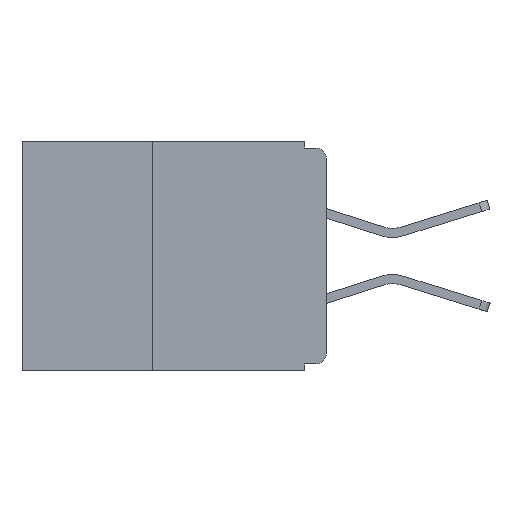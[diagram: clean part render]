
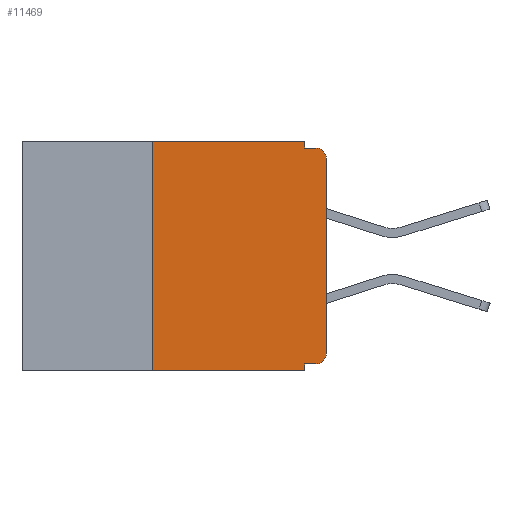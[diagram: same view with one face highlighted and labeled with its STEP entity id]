
A CAD part, left-side view. The second image highlights one B-rep face of the part: STEP entity #11469.
In plain terms, the highlighted planar face has unit normal (-1, 0, 0).
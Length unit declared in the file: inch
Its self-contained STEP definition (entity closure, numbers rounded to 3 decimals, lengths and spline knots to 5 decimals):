
#97 = DIRECTION ( 'NONE',  ( 0., 0., -1. ) ) ;
#202 = VERTEX_POINT ( 'NONE', #6253 ) ;
#437 = ORIENTED_EDGE ( 'NONE', *, *, #6418, .T. ) ;
#735 = ORIENTED_EDGE ( 'NONE', *, *, #865, .F. ) ;
#755 = EDGE_CURVE ( 'NONE', #5003, #202, #6537, .T. ) ;
#865 = EDGE_CURVE ( 'NONE', #6815, #7653, #2872, .T. ) ;
#989 = ORIENTED_EDGE ( 'NONE', *, *, #2569, .F. ) ;
#1243 = DIRECTION ( 'NONE',  ( 0., 0., -1. ) ) ;
#1258 = DIRECTION ( 'NONE',  ( 0., 0., -1. ) ) ;
#1265 = DIRECTION ( 'NONE',  ( -1., 0., 0. ) ) ;
#1297 = CARTESIAN_POINT ( 'NONE',  ( 0., 0.015, -0.305 ) ) ;
#1973 = CARTESIAN_POINT ( 'NONE',  ( 0., 0.031, -0.32 ) ) ;
#2001 = LINE ( 'NONE', #6248, #15230 ) ;
#2160 = CARTESIAN_POINT ( 'NONE',  ( 0., 0., -0.025 ) ) ;
#2253 = VERTEX_POINT ( 'NONE', #12908 ) ;
#2569 = EDGE_CURVE ( 'NONE', #202, #6815, #14484, .T. ) ;
#2672 = DIRECTION ( 'NONE',  ( 0., 0., -1. ) ) ;
#2676 = DIRECTION ( 'NONE',  ( -1., 0., 0. ) ) ;
#2709 = CARTESIAN_POINT ( 'NONE',  ( 0., 0.015, -0.025 ) ) ;
#2716 = VERTEX_POINT ( 'NONE', #4780 ) ;
#2820 = EDGE_CURVE ( 'NONE', #8170, #13883, #4053, .T. ) ;
#2872 = LINE ( 'NONE', #11974, #12372 ) ;
#3170 = EDGE_CURVE ( 'NONE', #10497, #6174, #8728, .T. ) ;
#3363 = EDGE_CURVE ( 'NONE', #2716, #8170, #2001, .T. ) ;
#3446 = ORIENTED_EDGE ( 'NONE', *, *, #16279, .F. ) ;
#3542 = LINE ( 'NONE', #7378, #13412 ) ;
#3854 = ORIENTED_EDGE ( 'NONE', *, *, #2820, .T. ) ;
#4053 = CIRCLE ( 'NONE', #14632, 0.015 ) ;
#4158 = ORIENTED_EDGE ( 'NONE', *, *, #3363, .T. ) ;
#4285 = VECTOR ( 'NONE', #6397, 39.37008 ) ;
#4346 = CIRCLE ( 'NONE', #13509, 0.015 ) ;
#4554 = ORIENTED_EDGE ( 'NONE', *, *, #755, .F. ) ;
#4652 = EDGE_CURVE ( 'NONE', #7653, #13883, #7502, .T. ) ;
#4780 = CARTESIAN_POINT ( 'NONE',  ( 0., 0., -0.305 ) ) ;
#5003 = VERTEX_POINT ( 'NONE', #7643 ) ;
#5066 = EDGE_CURVE ( 'NONE', #5003, #6174, #3542, .T. ) ;
#5258 = VECTOR ( 'NONE', #9967, 39.37008 ) ;
#5495 = DIRECTION ( 'NONE',  ( 0., 0., 1. ) ) ;
#5847 = DIRECTION ( 'NONE',  ( 0., 0., 1. ) ) ;
#6110 = EDGE_LOOP ( 'NONE', ( #4158, #3854, #9976, #735, #989, #4554, #12641, #6891, #3446, #437 ) ) ;
#6174 = VERTEX_POINT ( 'NONE', #7459 ) ;
#6248 = CARTESIAN_POINT ( 'NONE',  ( 0., 0., 0. ) ) ;
#6253 = CARTESIAN_POINT ( 'NONE',  ( 0., 0.25, 0. ) ) ;
#6369 = AXIS2_PLACEMENT_3D ( 'NONE', #15498, #7948, #97 ) ;
#6397 = DIRECTION ( 'NONE',  ( 0., -1., 0. ) ) ;
#6418 = EDGE_CURVE ( 'NONE', #2253, #2716, #4346, .T. ) ;
#6537 = LINE ( 'NONE', #8583, #12885 ) ;
#6675 = PLANE ( 'NONE',  #6369 ) ;
#6729 = CARTESIAN_POINT ( 'NONE',  ( 0., 0.437, 0. ) ) ;
#6796 = DIRECTION ( 'NONE',  ( 0., -1., 0. ) ) ;
#6815 = VERTEX_POINT ( 'NONE', #14040 ) ;
#6891 = ORIENTED_EDGE ( 'NONE', *, *, #3170, .F. ) ;
#6950 = CARTESIAN_POINT ( 'NONE',  ( 0., 0.031, -0.01 ) ) ;
#7378 = CARTESIAN_POINT ( 'NONE',  ( 0., 0.437, -0.33 ) ) ;
#7459 = CARTESIAN_POINT ( 'NONE',  ( 0., 0.031, -0.33 ) ) ;
#7502 = LINE ( 'NONE', #11016, #13425 ) ;
#7643 = CARTESIAN_POINT ( 'NONE',  ( 0., 0.25, -0.33 ) ) ;
#7653 = VERTEX_POINT ( 'NONE', #6950 ) ;
#7948 = DIRECTION ( 'NONE',  ( 1., 0., 0. ) ) ;
#8170 = VERTEX_POINT ( 'NONE', #2160 ) ;
#8583 = CARTESIAN_POINT ( 'NONE',  ( 0., 0.25, -0.33 ) ) ;
#8665 = CARTESIAN_POINT ( 'NONE',  ( 0., 0., -0.32 ) ) ;
#8728 = LINE ( 'NONE', #15152, #15036 ) ;
#9504 = CARTESIAN_POINT ( 'NONE',  ( 0., 0.015, -0.01 ) ) ;
#9762 = FACE_OUTER_BOUND ( 'NONE', #6110, .T. ) ;
#9967 = DIRECTION ( 'NONE',  ( 0., 1., 0. ) ) ;
#9976 = ORIENTED_EDGE ( 'NONE', *, *, #4652, .F. ) ;
#10497 = VERTEX_POINT ( 'NONE', #1973 ) ;
#10978 = DIRECTION ( 'NONE',  ( 0., -1., 0. ) ) ;
#11016 = CARTESIAN_POINT ( 'NONE',  ( 0., 0., -0.01 ) ) ;
#11469 = ADVANCED_FACE ( 'NONE', ( #9762 ), #6675, .F. ) ;
#11974 = CARTESIAN_POINT ( 'NONE',  ( 0., 0.031, 0. ) ) ;
#12094 = LINE ( 'NONE', #8665, #5258 ) ;
#12372 = VECTOR ( 'NONE', #1258, 39.37008 ) ;
#12641 = ORIENTED_EDGE ( 'NONE', *, *, #5066, .T. ) ;
#12885 = VECTOR ( 'NONE', #5847, 39.37008 ) ;
#12908 = CARTESIAN_POINT ( 'NONE',  ( 0., 0.015, -0.32 ) ) ;
#13412 = VECTOR ( 'NONE', #6796, 39.37008 ) ;
#13425 = VECTOR ( 'NONE', #10978, 39.37008 ) ;
#13509 = AXIS2_PLACEMENT_3D ( 'NONE', #1297, #1265, #1243 ) ;
#13883 = VERTEX_POINT ( 'NONE', #9504 ) ;
#14040 = CARTESIAN_POINT ( 'NONE',  ( 0., 0.031, 0. ) ) ;
#14484 = LINE ( 'NONE', #6729, #4285 ) ;
#14632 = AXIS2_PLACEMENT_3D ( 'NONE', #2709, #2676, #2672 ) ;
#14928 = DIRECTION ( 'NONE',  ( 0., 0., -1. ) ) ;
#15036 = VECTOR ( 'NONE', #14928, 39.37008 ) ;
#15152 = CARTESIAN_POINT ( 'NONE',  ( 0., 0.031, -0.33 ) ) ;
#15230 = VECTOR ( 'NONE', #5495, 39.37008 ) ;
#15498 = CARTESIAN_POINT ( 'NONE',  ( 0., 0.437, 0. ) ) ;
#16279 = EDGE_CURVE ( 'NONE', #2253, #10497, #12094, .T. ) ;
